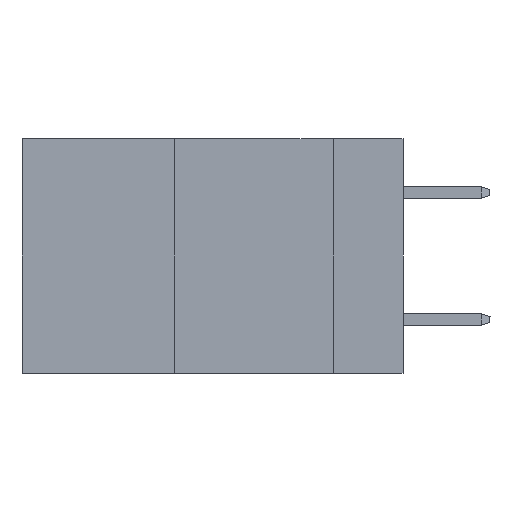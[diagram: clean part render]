
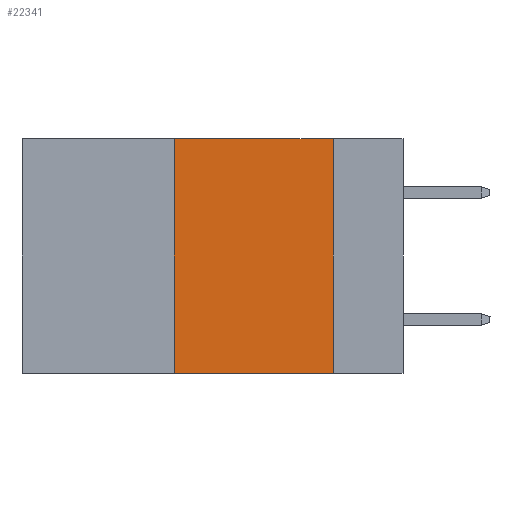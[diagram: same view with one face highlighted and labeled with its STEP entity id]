
A CAD part, left-side view. The second image highlights one B-rep face of the part: STEP entity #22341.
In plain terms, the highlighted planar face has unit normal (-1, 0, 0).
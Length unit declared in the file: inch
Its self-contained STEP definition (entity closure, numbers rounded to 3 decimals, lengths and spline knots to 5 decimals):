
#216 = DIRECTION ( 'NONE',  ( 0., 0., -1. ) ) ;
#217 = DIRECTION ( 'NONE',  ( 0., -1., 0. ) ) ;
#590 = PLANE ( 'NONE',  #31550 ) ;
#714 = VERTEX_POINT ( 'NONE', #21622 ) ;
#758 = EDGE_CURVE ( 'NONE', #33350, #19193, #24155, .T. ) ;
#1005 = EDGE_LOOP ( 'NONE', ( #19394, #22982, #19300, #27234 ) ) ;
#2326 = VERTEX_POINT ( 'NONE', #34290 ) ;
#5506 = LINE ( 'NONE', #11158, #33078 ) ;
#6272 = LINE ( 'NONE', #24329, #37455 ) ;
#9779 = FACE_OUTER_BOUND ( 'NONE', #1005, .T. ) ;
#11158 = CARTESIAN_POINT ( 'NONE',  ( 0., 0.11, 0. ) ) ;
#15009 = EDGE_CURVE ( 'NONE', #33350, #2326, #27107, .T. ) ;
#15535 = CARTESIAN_POINT ( 'NONE',  ( 0., 0.36, -0.37 ) ) ;
#17024 = EDGE_CURVE ( 'NONE', #19193, #714, #6272, .T. ) ;
#18696 = CARTESIAN_POINT ( 'NONE',  ( 0., 0.6, 0. ) ) ;
#18910 = CARTESIAN_POINT ( 'NONE',  ( 0., 0.36, 0. ) ) ;
#19193 = VERTEX_POINT ( 'NONE', #25778 ) ;
#19300 = ORIENTED_EDGE ( 'NONE', *, *, #758, .F. ) ;
#19394 = ORIENTED_EDGE ( 'NONE', *, *, #37745, .F. ) ;
#21622 = CARTESIAN_POINT ( 'NONE',  ( 0., 0.11, 0. ) ) ;
#22341 = ADVANCED_FACE ( 'NONE', ( #9779 ), #590, .F. ) ;
#22982 = ORIENTED_EDGE ( 'NONE', *, *, #17024, .F. ) ;
#24155 = LINE ( 'NONE', #18910, #27735 ) ;
#24329 = CARTESIAN_POINT ( 'NONE',  ( 0., 0.6, 0. ) ) ;
#25778 = CARTESIAN_POINT ( 'NONE',  ( 0., 0.36, 0. ) ) ;
#27107 = LINE ( 'NONE', #27305, #28986 ) ;
#27234 = ORIENTED_EDGE ( 'NONE', *, *, #15009, .T. ) ;
#27305 = CARTESIAN_POINT ( 'NONE',  ( 0., 0.6, -0.37 ) ) ;
#27439 = DIRECTION ( 'NONE',  ( 1., 0., 0. ) ) ;
#27735 = VECTOR ( 'NONE', #33682, 39.37008 ) ;
#28986 = VECTOR ( 'NONE', #35676, 39.37008 ) ;
#29226 = DIRECTION ( 'NONE',  ( 0., 0., -1. ) ) ;
#31550 = AXIS2_PLACEMENT_3D ( 'NONE', #18696, #27439, #216 ) ;
#33078 = VECTOR ( 'NONE', #29226, 39.37008 ) ;
#33350 = VERTEX_POINT ( 'NONE', #15535 ) ;
#33682 = DIRECTION ( 'NONE',  ( 0., 0., 1. ) ) ;
#34290 = CARTESIAN_POINT ( 'NONE',  ( 0., 0.11, -0.37 ) ) ;
#35676 = DIRECTION ( 'NONE',  ( 0., -1., 0. ) ) ;
#37455 = VECTOR ( 'NONE', #217, 39.37008 ) ;
#37745 = EDGE_CURVE ( 'NONE', #714, #2326, #5506, .T. ) ;
